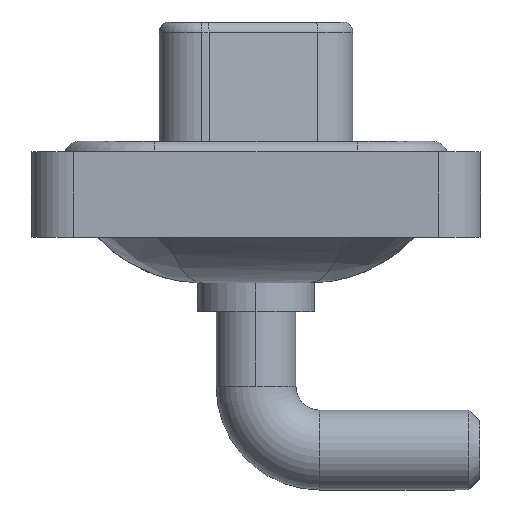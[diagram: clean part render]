
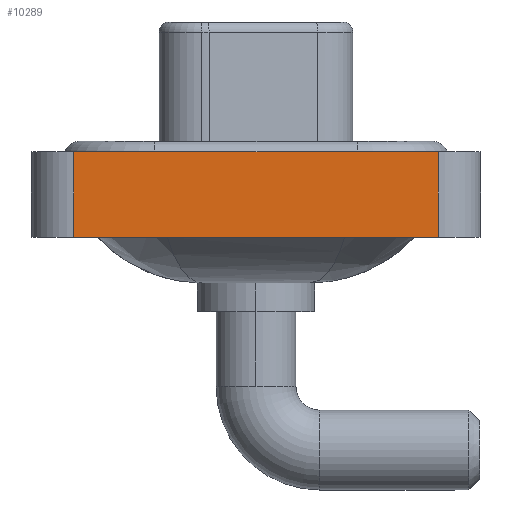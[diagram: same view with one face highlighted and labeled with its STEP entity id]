
A CAD part, left-side view. The second image highlights one B-rep face of the part: STEP entity #10289.
In plain terms, the highlighted planar face has unit normal (-1, 0, 0).
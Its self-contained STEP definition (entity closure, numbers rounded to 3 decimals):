
#587 = DIRECTION ( 'NONE',  ( -1., 0., 0. ) ) ;
#1006 = DIRECTION ( 'NONE',  ( 0., 0., 1. ) ) ;
#1600 = ORIENTED_EDGE ( 'NONE', *, *, #16916, .T. ) ;
#1640 = LINE ( 'NONE', #11001, #8780 ) ;
#1734 = EDGE_CURVE ( 'NONE', #7943, #4505, #1640, .T. ) ;
#1999 = ORIENTED_EDGE ( 'NONE', *, *, #11264, .F. ) ;
#3013 = CARTESIAN_POINT ( 'NONE',  ( -7.25, -8.55, -3.6 ) ) ;
#3215 = CARTESIAN_POINT ( 'NONE',  ( -7.25, 8.55, 0.4 ) ) ;
#4069 = ORIENTED_EDGE ( 'NONE', *, *, #7631, .T. ) ;
#4147 = VECTOR ( 'NONE', #1006, 1000. ) ;
#4505 = VERTEX_POINT ( 'NONE', #5486 ) ;
#5486 = CARTESIAN_POINT ( 'NONE',  ( -7.25, -8.55, 0.4 ) ) ;
#6734 = CARTESIAN_POINT ( 'NONE',  ( -7.25, -8.55, -3.6 ) ) ;
#7631 = EDGE_CURVE ( 'NONE', #12712, #11245, #12890, .T. ) ;
#7943 = VERTEX_POINT ( 'NONE', #3215 ) ;
#8194 = CARTESIAN_POINT ( 'NONE',  ( -7.25, 8.55, -3.6 ) ) ;
#8580 = DIRECTION ( 'NONE',  ( 0., 0., 1. ) ) ;
#8780 = VECTOR ( 'NONE', #12705, 1000. ) ;
#9230 = CARTESIAN_POINT ( 'NONE',  ( -7.25, -8.55, -3.6 ) ) ;
#10004 = CARTESIAN_POINT ( 'NONE',  ( -7.25, -8.55, -3.6 ) ) ;
#10289 = ADVANCED_FACE ( 'NONE', ( #16092 ), #11830, .T. ) ;
#10623 = VECTOR ( 'NONE', #8580, 1000. ) ;
#10941 = EDGE_LOOP ( 'NONE', ( #1600, #12645, #1999, #4069 ) ) ;
#11001 = CARTESIAN_POINT ( 'NONE',  ( -7.25, -8.55, 0.4 ) ) ;
#11245 = VERTEX_POINT ( 'NONE', #6734 ) ;
#11264 = EDGE_CURVE ( 'NONE', #12712, #7943, #13431, .T. ) ;
#11830 = PLANE ( 'NONE',  #16906 ) ;
#12645 = ORIENTED_EDGE ( 'NONE', *, *, #1734, .F. ) ;
#12705 = DIRECTION ( 'NONE',  ( 0., -1., 0. ) ) ;
#12712 = VERTEX_POINT ( 'NONE', #14074 ) ;
#12890 = LINE ( 'NONE', #10004, #13746 ) ;
#13431 = LINE ( 'NONE', #8194, #4147 ) ;
#13746 = VECTOR ( 'NONE', #16968, 1000. ) ;
#13821 = LINE ( 'NONE', #3013, #10623 ) ;
#14074 = CARTESIAN_POINT ( 'NONE',  ( -7.25, 8.55, -3.6 ) ) ;
#14734 = DIRECTION ( 'NONE',  ( 0., 0., 1. ) ) ;
#16092 = FACE_OUTER_BOUND ( 'NONE', #10941, .T. ) ;
#16906 = AXIS2_PLACEMENT_3D ( 'NONE', #9230, #587, #14734 ) ;
#16916 = EDGE_CURVE ( 'NONE', #11245, #4505, #13821, .T. ) ;
#16968 = DIRECTION ( 'NONE',  ( 0., -1., 0. ) ) ;
